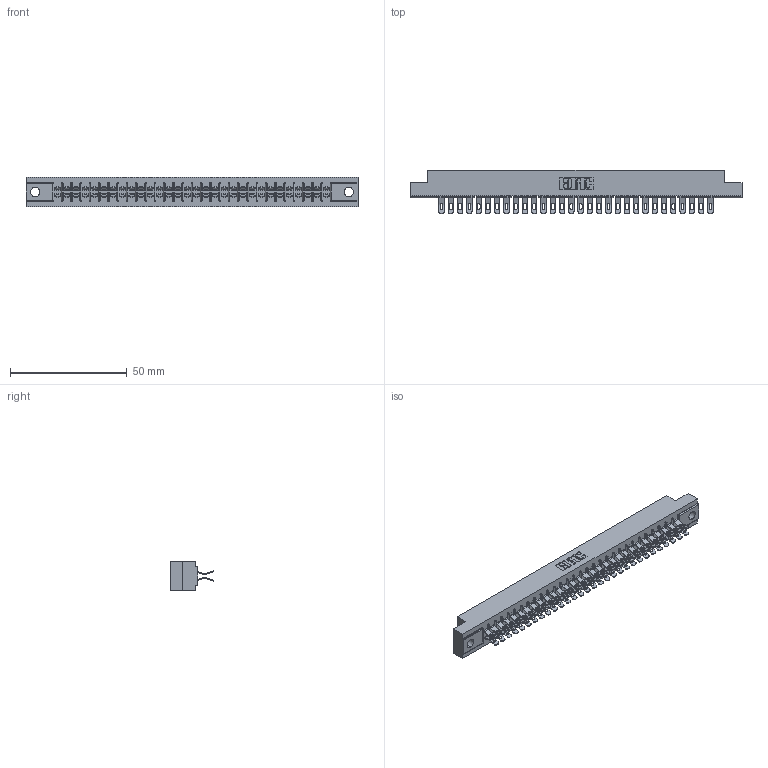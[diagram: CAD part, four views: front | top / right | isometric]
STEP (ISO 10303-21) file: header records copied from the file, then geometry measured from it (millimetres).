
FILE_DESCRIPTION (( 'STEP AP203' ), '1' );
FILE_NAME ('305-060-555-504.STEP', '2019-09-10T01:23:56', ( '' ), ( '' ), 'SwSTEP 2.0', 'SolidWorks 2016', '' );
FILE_SCHEMA (( 'CONFIG_CONTROL_DESIGN' ));
Length unit declared in the file: inch
Products named in the file (3): 305 Part_.156 Dia; 305-290-001_555; 305-060-555-504
Assembly tree (61 placements, depth 2):
  305-060-555-504
    305 Part_.156 Dia
    305-290-001_555  x60
Bounding box: 141.88 x 18.41 x 12.7 mm (x, y, z)
Volume: 14385.4 mm3; surface area: 19661.8 mm2
Topology: 61 solids, 61 shells, 4090 faces, 12202 edges, 7972 vertices
Faces by surface type: plane 2002, cylinder 1968, sphere 120
Entity records: 34985 total; most frequent: CARTESIAN_POINT 5812, ORIENTED_EDGE 5756, DIRECTION 5618, EDGE_CURVE 2878, VECTOR 2302, LINE 2302, VERTEX_POINT 1836, AXIS2_PLACEMENT_3D 1658
